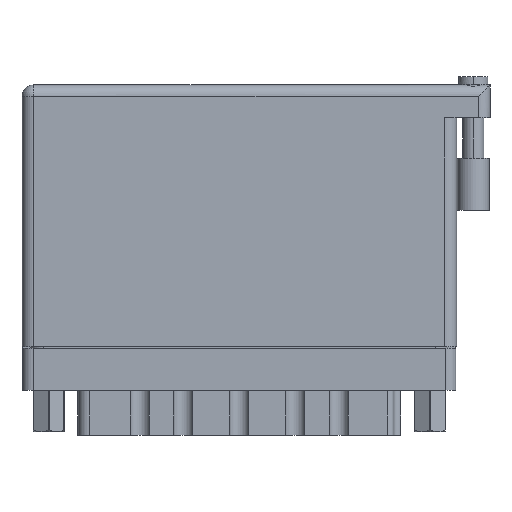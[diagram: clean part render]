
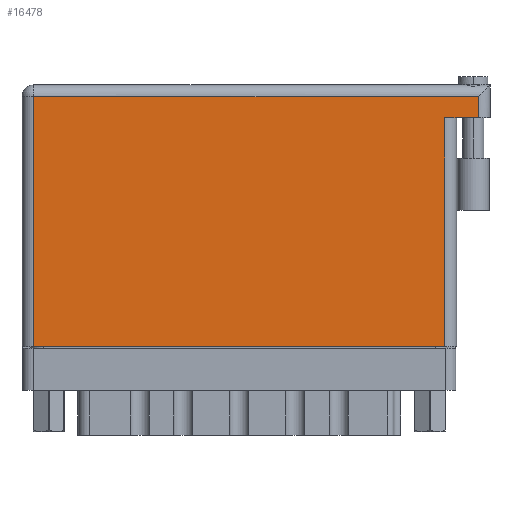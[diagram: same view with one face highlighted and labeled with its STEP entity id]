
A CAD part, front view. The second image highlights one B-rep face of the part: STEP entity #16478.
In plain terms, the highlighted face is planar.
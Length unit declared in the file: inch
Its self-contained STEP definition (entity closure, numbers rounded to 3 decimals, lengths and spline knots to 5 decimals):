
#398 = VERTEX_POINT ( 'NONE', #61850 ) ;
#1301 = LINE ( 'NONE', #28924, #4923 ) ;
#2086 = ORIENTED_EDGE ( 'NONE', *, *, #35198, .T. ) ;
#4258 = CARTESIAN_POINT ( 'NONE',  ( 0.07, 0., 0. ) ) ;
#4923 = VECTOR ( 'NONE', #20442, 39.37008 ) ;
#5497 = ORIENTED_EDGE ( 'NONE', *, *, #7182, .T. ) ;
#5743 = CARTESIAN_POINT ( 'NONE',  ( 2.73, 1.496, 0. ) ) ;
#7105 = AXIS2_PLACEMENT_3D ( 'NONE', #21619, #60506, #26619 ) ;
#7182 = EDGE_CURVE ( 'NONE', #39409, #19414, #38356, .T. ) ;
#7453 = EDGE_CURVE ( 'NONE', #398, #45796, #1301, .T. ) ;
#10791 = DIRECTION ( 'NONE',  ( 0., 1., 0. ) ) ;
#12949 = ORIENTED_EDGE ( 'NONE', *, *, #17206, .T. ) ;
#15189 = CARTESIAN_POINT ( 'NONE',  ( 2.53, 0., 0. ) ) ;
#15378 = VECTOR ( 'NONE', #21961, 39.37008 ) ;
#15809 = LINE ( 'NONE', #49647, #22748 ) ;
#16165 = CARTESIAN_POINT ( 'NONE',  ( 2.53, 1.369, 0. ) ) ;
#16478 = ADVANCED_FACE ( 'NONE', ( #26018 ), #46097, .F. ) ;
#17206 = EDGE_CURVE ( 'NONE', #33668, #39409, #56075, .T. ) ;
#17573 = CARTESIAN_POINT ( 'NONE',  ( 0., 1.496, 0. ) ) ;
#19414 = VERTEX_POINT ( 'NONE', #15189 ) ;
#20442 = DIRECTION ( 'NONE',  ( -1., 0., 0. ) ) ;
#21619 = CARTESIAN_POINT ( 'NONE',  ( 0., 1.566, 0. ) ) ;
#21961 = DIRECTION ( 'NONE',  ( -1., 0., 0. ) ) ;
#22748 = VECTOR ( 'NONE', #10791, 39.37008 ) ;
#23398 = DIRECTION ( 'NONE',  ( 0., -1., 0. ) ) ;
#24638 = CARTESIAN_POINT ( 'NONE',  ( 0.07, 1.496, 0. ) ) ;
#24919 = VECTOR ( 'NONE', #43069, 39.37008 ) ;
#25877 = DIRECTION ( 'NONE',  ( 0., 1., 0. ) ) ;
#26018 = FACE_OUTER_BOUND ( 'NONE', #31493, .T. ) ;
#26619 = DIRECTION ( 'NONE',  ( -1., 0., 0. ) ) ;
#26684 = VERTEX_POINT ( 'NONE', #5743 ) ;
#28132 = EDGE_CURVE ( 'NONE', #398, #26684, #15809, .T. ) ;
#28924 = CARTESIAN_POINT ( 'NONE',  ( 2.8, 1.369, 0. ) ) ;
#29224 = VECTOR ( 'NONE', #23398, 39.37008 ) ;
#30955 = ORIENTED_EDGE ( 'NONE', *, *, #7453, .F. ) ;
#31493 = EDGE_LOOP ( 'NONE', ( #5497, #44269, #30955, #51783, #2086, #12949 ) ) ;
#33454 = LINE ( 'NONE', #17573, #15378 ) ;
#33668 = VERTEX_POINT ( 'NONE', #24638 ) ;
#34034 = EDGE_CURVE ( 'NONE', #19414, #45796, #60364, .T. ) ;
#35198 = EDGE_CURVE ( 'NONE', #26684, #33668, #33454, .T. ) ;
#35602 = CARTESIAN_POINT ( 'NONE',  ( 2.53, 1.369, 0. ) ) ;
#38356 = LINE ( 'NONE', #57477, #24919 ) ;
#39409 = VERTEX_POINT ( 'NONE', #42710 ) ;
#42710 = CARTESIAN_POINT ( 'NONE',  ( 0.07, 0., 0. ) ) ;
#43069 = DIRECTION ( 'NONE',  ( 1., 0., 0. ) ) ;
#44269 = ORIENTED_EDGE ( 'NONE', *, *, #34034, .T. ) ;
#45367 = VECTOR ( 'NONE', #25877, 39.37008 ) ;
#45796 = VERTEX_POINT ( 'NONE', #16165 ) ;
#46097 = PLANE ( 'NONE',  #7105 ) ;
#49647 = CARTESIAN_POINT ( 'NONE',  ( 2.73, 1.566, 0. ) ) ;
#51783 = ORIENTED_EDGE ( 'NONE', *, *, #28132, .T. ) ;
#56075 = LINE ( 'NONE', #4258, #29224 ) ;
#57477 = CARTESIAN_POINT ( 'NONE',  ( 0., 0., 0. ) ) ;
#60364 = LINE ( 'NONE', #35602, #45367 ) ;
#60506 = DIRECTION ( 'NONE',  ( 0., 0., -1. ) ) ;
#61850 = CARTESIAN_POINT ( 'NONE',  ( 2.73, 1.369, 0. ) ) ;
